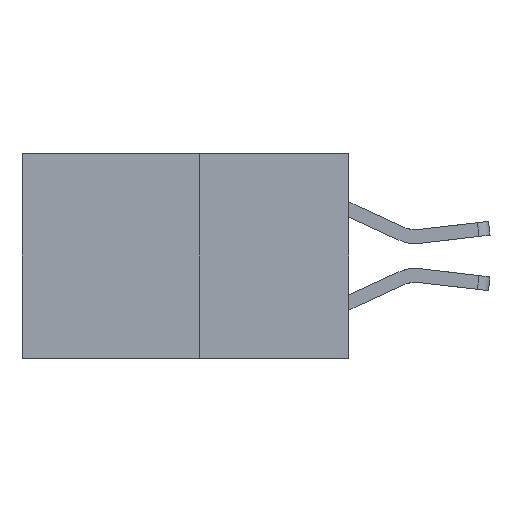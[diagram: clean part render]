
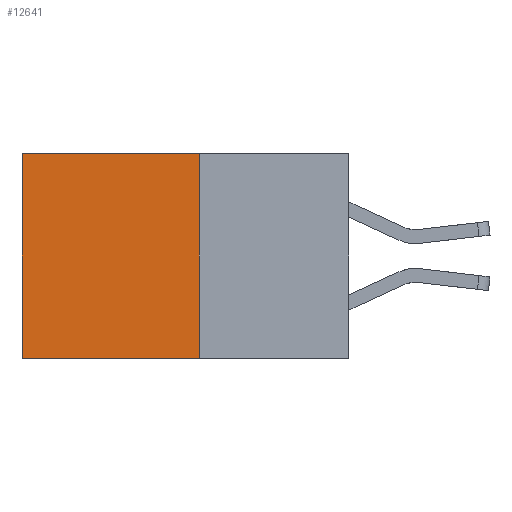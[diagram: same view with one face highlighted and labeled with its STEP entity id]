
A CAD part, left-side view. The second image highlights one B-rep face of the part: STEP entity #12641.
In plain terms, the highlighted planar face has unit normal (-1, 0, 0).
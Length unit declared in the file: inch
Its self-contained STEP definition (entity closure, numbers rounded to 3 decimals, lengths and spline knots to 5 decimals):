
#183 = ORIENTED_EDGE ( 'NONE', *, *, #4045, .T. ) ;
#352 = DIRECTION ( 'NONE',  ( 0., 1., 0. ) ) ;
#372 = CARTESIAN_POINT ( 'NONE',  ( 0.277, 0.27, 0. ) ) ;
#707 = DIRECTION ( 'NONE',  ( 0., 0., -1. ) ) ;
#936 = VECTOR ( 'NONE', #2809, 39.37008 ) ;
#1008 = CARTESIAN_POINT ( 'NONE',  ( 0.277, 0.27, 0. ) ) ;
#1091 = VECTOR ( 'NONE', #707, 39.37008 ) ;
#1574 = LINE ( 'NONE', #372, #12597 ) ;
#1909 = DIRECTION ( 'NONE',  ( 1., 0., 0. ) ) ;
#2432 = VERTEX_POINT ( 'NONE', #1008 ) ;
#2485 = EDGE_CURVE ( 'NONE', #4205, #4227, #4012, .T. ) ;
#2809 = DIRECTION ( 'NONE',  ( 0., 1., 0. ) ) ;
#3838 = CARTESIAN_POINT ( 'NONE',  ( 0.277, 0.59, 0. ) ) ;
#3991 = ORIENTED_EDGE ( 'NONE', *, *, #9945, .F. ) ;
#4012 = LINE ( 'NONE', #7961, #1091 ) ;
#4045 = EDGE_CURVE ( 'NONE', #2432, #4205, #1574, .T. ) ;
#4205 = VERTEX_POINT ( 'NONE', #3838 ) ;
#4227 = VERTEX_POINT ( 'NONE', #9026 ) ;
#4595 = LINE ( 'NONE', #11832, #7374 ) ;
#5165 = PLANE ( 'NONE',  #10119 ) ;
#5225 = ORIENTED_EDGE ( 'NONE', *, *, #11842, .F. ) ;
#5825 = DIRECTION ( 'NONE',  ( 0., 0., -1. ) ) ;
#7374 = VECTOR ( 'NONE', #5825, 39.37008 ) ;
#7607 = FACE_OUTER_BOUND ( 'NONE', #10724, .T. ) ;
#7961 = CARTESIAN_POINT ( 'NONE',  ( 0.277, 0.59, -0.37 ) ) ;
#8241 = CARTESIAN_POINT ( 'NONE',  ( 0.277, 0.27, -0.37 ) ) ;
#9025 = LINE ( 'NONE', #10016, #936 ) ;
#9026 = CARTESIAN_POINT ( 'NONE',  ( 0.277, 0.59, -0.37 ) ) ;
#9224 = DIRECTION ( 'NONE',  ( 0., 0., -1. ) ) ;
#9444 = VERTEX_POINT ( 'NONE', #11988 ) ;
#9945 = EDGE_CURVE ( 'NONE', #2432, #9444, #4595, .T. ) ;
#10016 = CARTESIAN_POINT ( 'NONE',  ( 0.277, 0.27, -0.37 ) ) ;
#10119 = AXIS2_PLACEMENT_3D ( 'NONE', #8241, #1909, #9224 ) ;
#10724 = EDGE_LOOP ( 'NONE', ( #11461, #5225, #3991, #183 ) ) ;
#11461 = ORIENTED_EDGE ( 'NONE', *, *, #2485, .T. ) ;
#11832 = CARTESIAN_POINT ( 'NONE',  ( 0.277, 0.27, -0.37 ) ) ;
#11842 = EDGE_CURVE ( 'NONE', #9444, #4227, #9025, .T. ) ;
#11988 = CARTESIAN_POINT ( 'NONE',  ( 0.277, 0.27, -0.37 ) ) ;
#12597 = VECTOR ( 'NONE', #352, 39.37008 ) ;
#12641 = ADVANCED_FACE ( 'NONE', ( #7607 ), #5165, .F. ) ;
